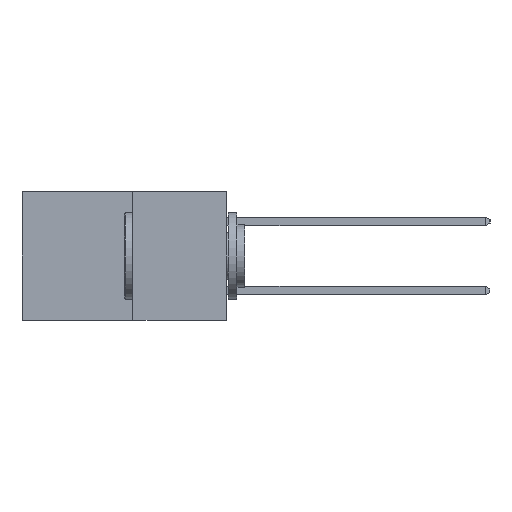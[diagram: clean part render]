
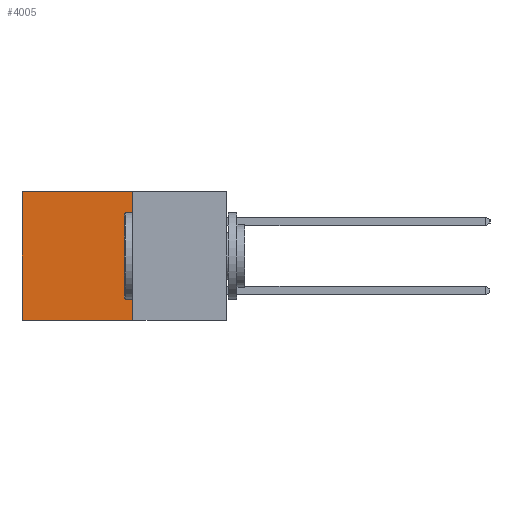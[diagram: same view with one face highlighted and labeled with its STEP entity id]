
A CAD part, left-side view. The second image highlights one B-rep face of the part: STEP entity #4005.
In plain terms, the highlighted planar face has unit normal (-1, 0, 0).
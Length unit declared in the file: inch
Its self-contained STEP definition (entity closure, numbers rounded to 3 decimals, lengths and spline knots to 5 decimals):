
#39 = EDGE_CURVE ( 'NONE', #6711, #6788, #2923, .T. ) ;
#875 = DIRECTION ( 'NONE',  ( 0., 1., 0. ) ) ;
#1015 = CARTESIAN_POINT ( 'NONE',  ( 0.277, 0.27, 0. ) ) ;
#1288 = ORIENTED_EDGE ( 'NONE', *, *, #4350, .T. ) ;
#1555 = FACE_OUTER_BOUND ( 'NONE', #6586, .T. ) ;
#1666 = EDGE_CURVE ( 'NONE', #6788, #2970, #7566, .T. ) ;
#2631 = VECTOR ( 'NONE', #5733, 39.37008 ) ;
#2923 = LINE ( 'NONE', #5736, #2631 ) ;
#2970 = VERTEX_POINT ( 'NONE', #5658 ) ;
#3460 = LINE ( 'NONE', #7799, #6035 ) ;
#3961 = AXIS2_PLACEMENT_3D ( 'NONE', #9713, #9609, #9591 ) ;
#4005 = ADVANCED_FACE ( 'NONE', ( #1555 ), #9628, .F. ) ;
#4350 = EDGE_CURVE ( 'NONE', #8316, #2970, #3460, .T. ) ;
#5309 = LINE ( 'NONE', #1015, #7510 ) ;
#5378 = ORIENTED_EDGE ( 'NONE', *, *, #8075, .T. ) ;
#5658 = CARTESIAN_POINT ( 'NONE',  ( 0.277, 0.59, -0.37 ) ) ;
#5733 = DIRECTION ( 'NONE',  ( 0., 0., -1. ) ) ;
#5736 = CARTESIAN_POINT ( 'NONE',  ( 0.277, 0.27, -0.37 ) ) ;
#6035 = VECTOR ( 'NONE', #7833, 39.37008 ) ;
#6066 = CARTESIAN_POINT ( 'NONE',  ( 0.277, 0.27, -0.37 ) ) ;
#6273 = DIRECTION ( 'NONE',  ( 0., 1., 0. ) ) ;
#6586 = EDGE_LOOP ( 'NONE', ( #1288, #9140, #7014, #5378 ) ) ;
#6711 = VERTEX_POINT ( 'NONE', #10466 ) ;
#6788 = VERTEX_POINT ( 'NONE', #10291 ) ;
#6959 = CARTESIAN_POINT ( 'NONE',  ( 0.277, 0.59, 0. ) ) ;
#7014 = ORIENTED_EDGE ( 'NONE', *, *, #39, .F. ) ;
#7290 = VECTOR ( 'NONE', #6273, 39.37008 ) ;
#7510 = VECTOR ( 'NONE', #875, 39.37008 ) ;
#7566 = LINE ( 'NONE', #6066, #7290 ) ;
#7799 = CARTESIAN_POINT ( 'NONE',  ( 0.277, 0.59, -0.37 ) ) ;
#7833 = DIRECTION ( 'NONE',  ( 0., 0., -1. ) ) ;
#8075 = EDGE_CURVE ( 'NONE', #6711, #8316, #5309, .T. ) ;
#8316 = VERTEX_POINT ( 'NONE', #6959 ) ;
#9140 = ORIENTED_EDGE ( 'NONE', *, *, #1666, .F. ) ;
#9591 = DIRECTION ( 'NONE',  ( 0., 0., -1. ) ) ;
#9609 = DIRECTION ( 'NONE',  ( 1., 0., 0. ) ) ;
#9628 = PLANE ( 'NONE',  #3961 ) ;
#9713 = CARTESIAN_POINT ( 'NONE',  ( 0.277, 0.27, -0.37 ) ) ;
#10291 = CARTESIAN_POINT ( 'NONE',  ( 0.277, 0.27, -0.37 ) ) ;
#10466 = CARTESIAN_POINT ( 'NONE',  ( 0.277, 0.27, 0. ) ) ;
